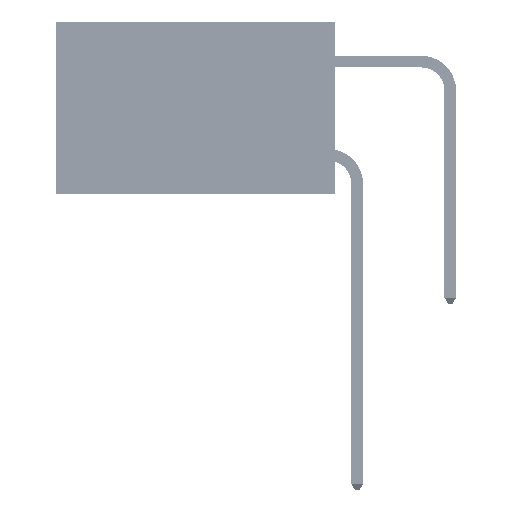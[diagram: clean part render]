
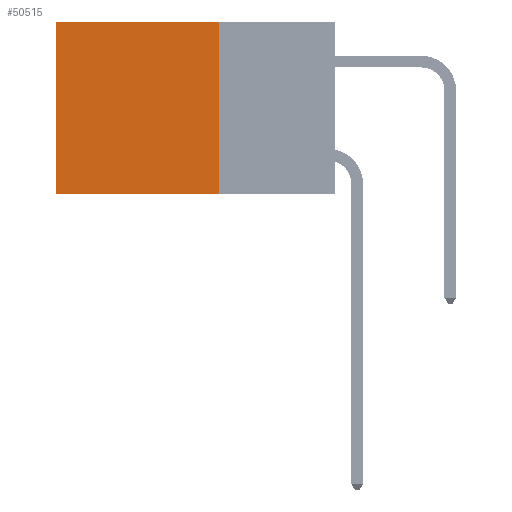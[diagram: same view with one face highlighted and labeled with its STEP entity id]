
A CAD part, left-side view. The second image highlights one B-rep face of the part: STEP entity #50515.
In plain terms, the highlighted planar face has unit normal (-1, 0, 0).
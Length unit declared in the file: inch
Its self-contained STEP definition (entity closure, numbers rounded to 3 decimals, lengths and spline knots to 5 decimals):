
#3117 = VERTEX_POINT ( 'NONE', #45929 ) ;
#3625 = CARTESIAN_POINT ( 'NONE',  ( 0.2875, 0.25, 0. ) ) ;
#4048 = DIRECTION ( 'NONE',  ( 0., 0., -1. ) ) ;
#5611 = CARTESIAN_POINT ( 'NONE',  ( 0.2875, 0.6, 0. ) ) ;
#5916 = ORIENTED_EDGE ( 'NONE', *, *, #15376, .T. ) ;
#7031 = VECTOR ( 'NONE', #20242, 39.37008 ) ;
#7466 = PLANE ( 'NONE',  #16894 ) ;
#9247 = ORIENTED_EDGE ( 'NONE', *, *, #12543, .T. ) ;
#10291 = LINE ( 'NONE', #41519, #15383 ) ;
#11979 = VERTEX_POINT ( 'NONE', #50448 ) ;
#12543 = EDGE_CURVE ( 'NONE', #12670, #3117, #17566, .T. ) ;
#12670 = VERTEX_POINT ( 'NONE', #5611 ) ;
#15376 = EDGE_CURVE ( 'NONE', #11979, #12670, #35797, .T. ) ;
#15383 = VECTOR ( 'NONE', #33164, 39.37008 ) ;
#15580 = DIRECTION ( 'NONE',  ( 0., 1., 0. ) ) ;
#16894 = AXIS2_PLACEMENT_3D ( 'NONE', #26598, #24605, #4048 ) ;
#17566 = LINE ( 'NONE', #49330, #30317 ) ;
#20242 = DIRECTION ( 'NONE',  ( 0., 1., 0. ) ) ;
#20879 = EDGE_CURVE ( 'NONE', #11979, #45701, #10291, .T. ) ;
#21582 = LINE ( 'NONE', #35909, #40051 ) ;
#24605 = DIRECTION ( 'NONE',  ( 1., 0., 0. ) ) ;
#26047 = FACE_OUTER_BOUND ( 'NONE', #51685, .T. ) ;
#26598 = CARTESIAN_POINT ( 'NONE',  ( 0.2875, 0.25, 0. ) ) ;
#29007 = DIRECTION ( 'NONE',  ( 0., 0., -1. ) ) ;
#30195 = ORIENTED_EDGE ( 'NONE', *, *, #42723, .F. ) ;
#30317 = VECTOR ( 'NONE', #29007, 39.37008 ) ;
#33164 = DIRECTION ( 'NONE',  ( 0., 0., -1. ) ) ;
#35797 = LINE ( 'NONE', #3625, #7031 ) ;
#35909 = CARTESIAN_POINT ( 'NONE',  ( 0.2875, 0.25, -0.37 ) ) ;
#40051 = VECTOR ( 'NONE', #15580, 39.37008 ) ;
#41519 = CARTESIAN_POINT ( 'NONE',  ( 0.2875, 0.25, 0. ) ) ;
#42723 = EDGE_CURVE ( 'NONE', #45701, #3117, #21582, .T. ) ;
#45701 = VERTEX_POINT ( 'NONE', #48335 ) ;
#45929 = CARTESIAN_POINT ( 'NONE',  ( 0.2875, 0.6, -0.37 ) ) ;
#48335 = CARTESIAN_POINT ( 'NONE',  ( 0.2875, 0.25, -0.37 ) ) ;
#49330 = CARTESIAN_POINT ( 'NONE',  ( 0.2875, 0.6, 0. ) ) ;
#50014 = ORIENTED_EDGE ( 'NONE', *, *, #20879, .F. ) ;
#50448 = CARTESIAN_POINT ( 'NONE',  ( 0.2875, 0.25, 0. ) ) ;
#50515 = ADVANCED_FACE ( 'NONE', ( #26047 ), #7466, .F. ) ;
#51685 = EDGE_LOOP ( 'NONE', ( #9247, #30195, #50014, #5916 ) ) ;
